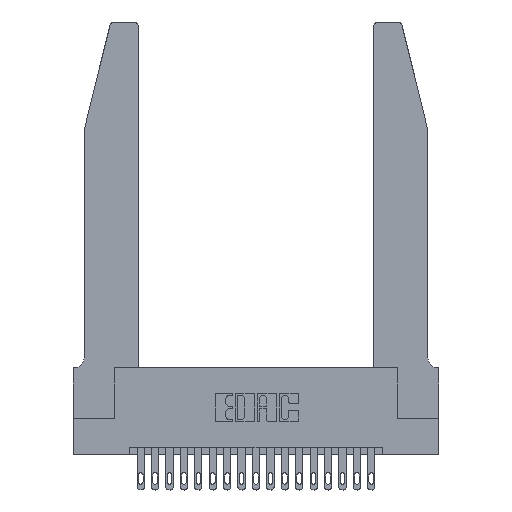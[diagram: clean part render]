
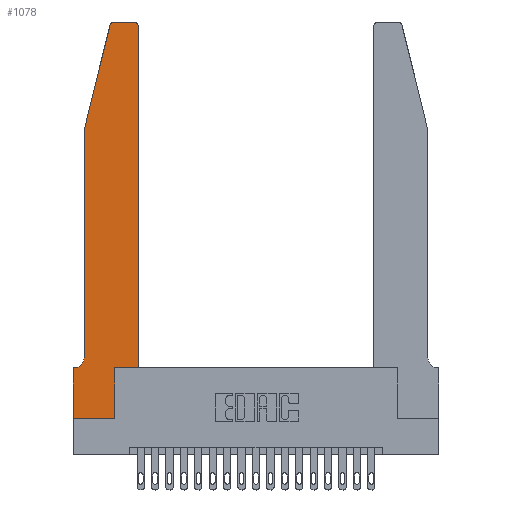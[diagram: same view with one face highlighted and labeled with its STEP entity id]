
A CAD part, top view. The second image highlights one B-rep face of the part: STEP entity #1078.
In plain terms, the highlighted planar face has unit normal (0, 0, 1).
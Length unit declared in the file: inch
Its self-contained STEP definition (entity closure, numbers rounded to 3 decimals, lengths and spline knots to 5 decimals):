
#80 = VECTOR ( 'NONE', #7949, 39.37008 ) ;
#450 = VECTOR ( 'NONE', #7582, 39.37008 ) ;
#573 = CARTESIAN_POINT ( 'NONE',  ( 0.4505, 0.35, 0.37 ) ) ;
#842 = VECTOR ( 'NONE', #5753, 39.37008 ) ;
#1036 = EDGE_CURVE ( 'NONE', #15831, #3769, #19485, .T. ) ;
#1078 = ADVANCED_FACE ( 'NONE', ( #12221 ), #14557, .T. ) ;
#1364 = DIRECTION ( 'NONE',  ( 1., 0., 0. ) ) ;
#1388 = ORIENTED_EDGE ( 'NONE', *, *, #6686, .T. ) ;
#1539 = EDGE_LOOP ( 'NONE', ( #15408, #18345, #5459, #5067, #1388, #21379, #10010, #14277, #2768, #19620, #19615, #18415 ) ) ;
#1608 = EDGE_CURVE ( 'NONE', #3726, #20988, #8837, .T. ) ;
#1701 = CARTESIAN_POINT ( 'NONE',  ( 0.0755, 0.35, 0.37 ) ) ;
#1847 = VERTEX_POINT ( 'NONE', #4610 ) ;
#2380 = CARTESIAN_POINT ( 'NONE',  ( 0.4505, 2.72, 0.37 ) ) ;
#2650 = CARTESIAN_POINT ( 'NONE',  ( 0.2865, 0.35, 0.37 ) ) ;
#2768 = ORIENTED_EDGE ( 'NONE', *, *, #6318, .T. ) ;
#2774 = CARTESIAN_POINT ( 'NONE',  ( 0.0755, 2., 0.37 ) ) ;
#3726 = VERTEX_POINT ( 'NONE', #2650 ) ;
#3769 = VERTEX_POINT ( 'NONE', #14164 ) ;
#4056 = EDGE_CURVE ( 'NONE', #20988, #8880, #16022, .T. ) ;
#4121 = CARTESIAN_POINT ( 'NONE',  ( 0.284, 2.75, 0.37 ) ) ;
#4393 = EDGE_CURVE ( 'NONE', #1847, #10351, #7693, .T. ) ;
#4606 = CARTESIAN_POINT ( 'NONE',  ( 0., 0.35, 0.37 ) ) ;
#4610 = CARTESIAN_POINT ( 'NONE',  ( 0.25487, 2.72718, 0.37 ) ) ;
#4657 = DIRECTION ( 'NONE',  ( 1., 0., 0. ) ) ;
#5067 = ORIENTED_EDGE ( 'NONE', *, *, #12960, .T. ) ;
#5459 = ORIENTED_EDGE ( 'NONE', *, *, #4393, .T. ) ;
#5497 = VERTEX_POINT ( 'NONE', #11088 ) ;
#5531 = CARTESIAN_POINT ( 'NONE',  ( 0.0755, 2., 0.37 ) ) ;
#5753 = DIRECTION ( 'NONE',  ( 1., 0., 0. ) ) ;
#5827 = DIRECTION ( 'NONE',  ( 0., 1., 0. ) ) ;
#5909 = CARTESIAN_POINT ( 'NONE',  ( 0.2865, 0.35, 0.37 ) ) ;
#6318 = EDGE_CURVE ( 'NONE', #20862, #3726, #18031, .T. ) ;
#6686 = EDGE_CURVE ( 'NONE', #9877, #8054, #8392, .T. ) ;
#6825 = DIRECTION ( 'NONE',  ( -1., 0., 0. ) ) ;
#7248 = VECTOR ( 'NONE', #1364, 39.37008 ) ;
#7302 = CARTESIAN_POINT ( 'NONE',  ( 0.0055, 0.35, 0.37 ) ) ;
#7376 = EDGE_CURVE ( 'NONE', #16183, #1847, #7586, .T. ) ;
#7582 = DIRECTION ( 'NONE',  ( -0.239, -0.971, 0. ) ) ;
#7586 = CIRCLE ( 'NONE', #12514, 0.03 ) ;
#7693 = LINE ( 'NONE', #5531, #450 ) ;
#7809 = CARTESIAN_POINT ( 'NONE',  ( 0., 0., 0.37 ) ) ;
#7949 = DIRECTION ( 'NONE',  ( 0., -1., 0. ) ) ;
#8054 = VERTEX_POINT ( 'NONE', #7302 ) ;
#8392 = CIRCLE ( 'NONE', #16999, 0.07 ) ;
#8599 = CARTESIAN_POINT ( 'NONE',  ( 0., 0.35, 0.37 ) ) ;
#8782 = LINE ( 'NONE', #7809, #7248 ) ;
#8837 = LINE ( 'NONE', #573, #842 ) ;
#8880 = VERTEX_POINT ( 'NONE', #2380 ) ;
#9841 = CARTESIAN_POINT ( 'NONE',  ( 0.2605, 2.75, 0.37 ) ) ;
#9877 = VERTEX_POINT ( 'NONE', #12987 ) ;
#10008 = EDGE_CURVE ( 'NONE', #8054, #15831, #14520, .T. ) ;
#10010 = ORIENTED_EDGE ( 'NONE', *, *, #1036, .T. ) ;
#10351 = VERTEX_POINT ( 'NONE', #10435 ) ;
#10435 = CARTESIAN_POINT ( 'NONE',  ( 0.0755, 2., 0.37 ) ) ;
#10746 = EDGE_CURVE ( 'NONE', #8880, #5497, #19392, .T. ) ;
#11088 = CARTESIAN_POINT ( 'NONE',  ( 0.4205, 2.75, 0.37 ) ) ;
#12221 = FACE_OUTER_BOUND ( 'NONE', #1539, .T. ) ;
#12514 = AXIS2_PLACEMENT_3D ( 'NONE', #17669, #14058, #17460 ) ;
#12932 = VECTOR ( 'NONE', #6825, 39.37008 ) ;
#12960 = EDGE_CURVE ( 'NONE', #10351, #9877, #18791, .T. ) ;
#12987 = CARTESIAN_POINT ( 'NONE',  ( 0.0755, 0.42, 0.37 ) ) ;
#13084 = VECTOR ( 'NONE', #5827, 39.37008 ) ;
#13274 = DIRECTION ( 'NONE',  ( -1., 0., 0. ) ) ;
#13454 = CARTESIAN_POINT ( 'NONE',  ( 0.0055, 0.42, 0.37 ) ) ;
#13530 = DIRECTION ( 'NONE',  ( -1., 0., 0. ) ) ;
#14058 = DIRECTION ( 'NONE',  ( 0., 0., 1. ) ) ;
#14164 = CARTESIAN_POINT ( 'NONE',  ( 0., 0., 0.37 ) ) ;
#14277 = ORIENTED_EDGE ( 'NONE', *, *, #19631, .T. ) ;
#14339 = CARTESIAN_POINT ( 'NONE',  ( 0., 0., 0.37 ) ) ;
#14520 = LINE ( 'NONE', #1701, #16811 ) ;
#14557 = PLANE ( 'NONE',  #17057 ) ;
#15408 = ORIENTED_EDGE ( 'NONE', *, *, #15737, .T. ) ;
#15737 = EDGE_CURVE ( 'NONE', #5497, #16183, #16346, .T. ) ;
#15831 = VERTEX_POINT ( 'NONE', #8599 ) ;
#15993 = DIRECTION ( 'NONE',  ( 0., -1., 0. ) ) ;
#16022 = LINE ( 'NONE', #20946, #18088 ) ;
#16183 = VERTEX_POINT ( 'NONE', #4121 ) ;
#16346 = LINE ( 'NONE', #9841, #12932 ) ;
#16811 = VECTOR ( 'NONE', #13274, 39.37008 ) ;
#16892 = CARTESIAN_POINT ( 'NONE',  ( 0.4205, 2.72, 0.37 ) ) ;
#16999 = AXIS2_PLACEMENT_3D ( 'NONE', #13454, #20111, #13530 ) ;
#17057 = AXIS2_PLACEMENT_3D ( 'NONE', #4606, #19460, #4657 ) ;
#17460 = DIRECTION ( 'NONE',  ( 1., 0., 0. ) ) ;
#17669 = CARTESIAN_POINT ( 'NONE',  ( 0.284, 2.72, 0.37 ) ) ;
#17704 = DIRECTION ( 'NONE',  ( 0., 1., 0. ) ) ;
#17841 = AXIS2_PLACEMENT_3D ( 'NONE', #16892, #19913, #18475 ) ;
#18031 = LINE ( 'NONE', #5909, #13084 ) ;
#18088 = VECTOR ( 'NONE', #17704, 39.37008 ) ;
#18345 = ORIENTED_EDGE ( 'NONE', *, *, #7376, .T. ) ;
#18415 = ORIENTED_EDGE ( 'NONE', *, *, #10746, .T. ) ;
#18475 = DIRECTION ( 'NONE',  ( 1., 0., 0. ) ) ;
#18791 = LINE ( 'NONE', #2774, #21407 ) ;
#19392 = CIRCLE ( 'NONE', #17841, 0.03 ) ;
#19460 = DIRECTION ( 'NONE',  ( 0., 0., 1. ) ) ;
#19485 = LINE ( 'NONE', #14339, #80 ) ;
#19615 = ORIENTED_EDGE ( 'NONE', *, *, #4056, .T. ) ;
#19620 = ORIENTED_EDGE ( 'NONE', *, *, #1608, .T. ) ;
#19631 = EDGE_CURVE ( 'NONE', #3769, #20862, #8782, .T. ) ;
#19913 = DIRECTION ( 'NONE',  ( 0., 0., 1. ) ) ;
#19947 = CARTESIAN_POINT ( 'NONE',  ( 0.4505, 0.35, 0.37 ) ) ;
#20111 = DIRECTION ( 'NONE',  ( 0., 0., -1. ) ) ;
#20862 = VERTEX_POINT ( 'NONE', #21262 ) ;
#20946 = CARTESIAN_POINT ( 'NONE',  ( 0.4505, 0.35, 0.37 ) ) ;
#20988 = VERTEX_POINT ( 'NONE', #19947 ) ;
#21262 = CARTESIAN_POINT ( 'NONE',  ( 0.2865, 0., 0.37 ) ) ;
#21379 = ORIENTED_EDGE ( 'NONE', *, *, #10008, .T. ) ;
#21407 = VECTOR ( 'NONE', #15993, 39.37008 ) ;
